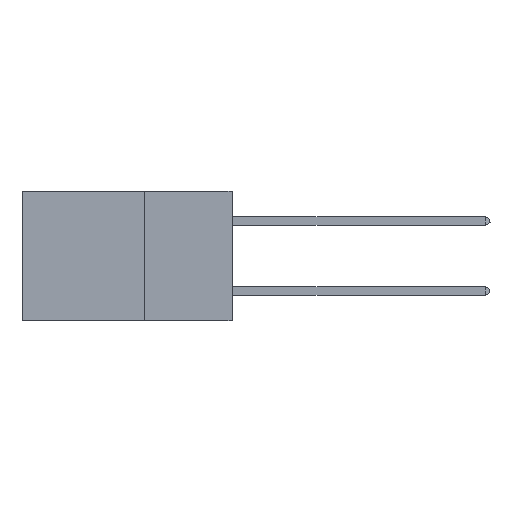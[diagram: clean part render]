
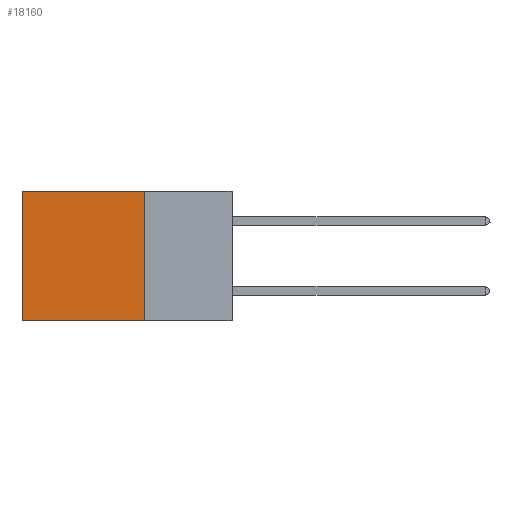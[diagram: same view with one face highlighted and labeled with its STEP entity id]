
A CAD part, left-side view. The second image highlights one B-rep face of the part: STEP entity #18160.
In plain terms, the highlighted planar face has unit normal (-1, 0, 0).
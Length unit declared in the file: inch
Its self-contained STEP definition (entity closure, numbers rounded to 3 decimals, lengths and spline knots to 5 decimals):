
#1509 = VERTEX_POINT ( 'NONE', #3529 ) ;
#1710 = DIRECTION ( 'NONE',  ( 0., 1., 0. ) ) ;
#3271 = CARTESIAN_POINT ( 'NONE',  ( 0.2875, 0.25, 0. ) ) ;
#3529 = CARTESIAN_POINT ( 'NONE',  ( 0.2875, 0.25, -0.37 ) ) ;
#7501 = CARTESIAN_POINT ( 'NONE',  ( 0.2875, 0.25, 0. ) ) ;
#8845 = LINE ( 'NONE', #14292, #20315 ) ;
#8854 = CARTESIAN_POINT ( 'NONE',  ( 0.2875, 0.6, 0. ) ) ;
#9717 = LINE ( 'NONE', #33075, #20730 ) ;
#11090 = VERTEX_POINT ( 'NONE', #24540 ) ;
#11987 = VERTEX_POINT ( 'NONE', #16849 ) ;
#12596 = LINE ( 'NONE', #7501, #33683 ) ;
#13162 = PLANE ( 'NONE',  #13643 ) ;
#13486 = EDGE_CURVE ( 'NONE', #18110, #11090, #9717, .T. ) ;
#13643 = AXIS2_PLACEMENT_3D ( 'NONE', #3271, #28968, #19437 ) ;
#14292 = CARTESIAN_POINT ( 'NONE',  ( 0.2875, 0.25, 0. ) ) ;
#16782 = FACE_OUTER_BOUND ( 'NONE', #18301, .T. ) ;
#16849 = CARTESIAN_POINT ( 'NONE',  ( 0.2875, 0.25, 0. ) ) ;
#18110 = VERTEX_POINT ( 'NONE', #8854 ) ;
#18160 = ADVANCED_FACE ( 'NONE', ( #16782 ), #13162, .F. ) ;
#18301 = EDGE_LOOP ( 'NONE', ( #33828, #19517, #26408, #34616 ) ) ;
#19437 = DIRECTION ( 'NONE',  ( 0., 0., -1. ) ) ;
#19517 = ORIENTED_EDGE ( 'NONE', *, *, #19892, .F. ) ;
#19892 = EDGE_CURVE ( 'NONE', #1509, #11090, #26822, .T. ) ;
#20315 = VECTOR ( 'NONE', #25885, 39.37008 ) ;
#20432 = DIRECTION ( 'NONE',  ( 0., 0., -1. ) ) ;
#20730 = VECTOR ( 'NONE', #20432, 39.37008 ) ;
#22178 = EDGE_CURVE ( 'NONE', #11987, #18110, #12596, .T. ) ;
#24178 = CARTESIAN_POINT ( 'NONE',  ( 0.2875, 0.25, -0.37 ) ) ;
#24348 = EDGE_CURVE ( 'NONE', #11987, #1509, #8845, .T. ) ;
#24540 = CARTESIAN_POINT ( 'NONE',  ( 0.2875, 0.6, -0.37 ) ) ;
#25885 = DIRECTION ( 'NONE',  ( 0., 0., -1. ) ) ;
#26408 = ORIENTED_EDGE ( 'NONE', *, *, #24348, .F. ) ;
#26822 = LINE ( 'NONE', #24178, #28537 ) ;
#26990 = DIRECTION ( 'NONE',  ( 0., 1., 0. ) ) ;
#28537 = VECTOR ( 'NONE', #26990, 39.37008 ) ;
#28968 = DIRECTION ( 'NONE',  ( 1., 0., 0. ) ) ;
#33075 = CARTESIAN_POINT ( 'NONE',  ( 0.2875, 0.6, 0. ) ) ;
#33683 = VECTOR ( 'NONE', #1710, 39.37008 ) ;
#33828 = ORIENTED_EDGE ( 'NONE', *, *, #13486, .T. ) ;
#34616 = ORIENTED_EDGE ( 'NONE', *, *, #22178, .T. ) ;
